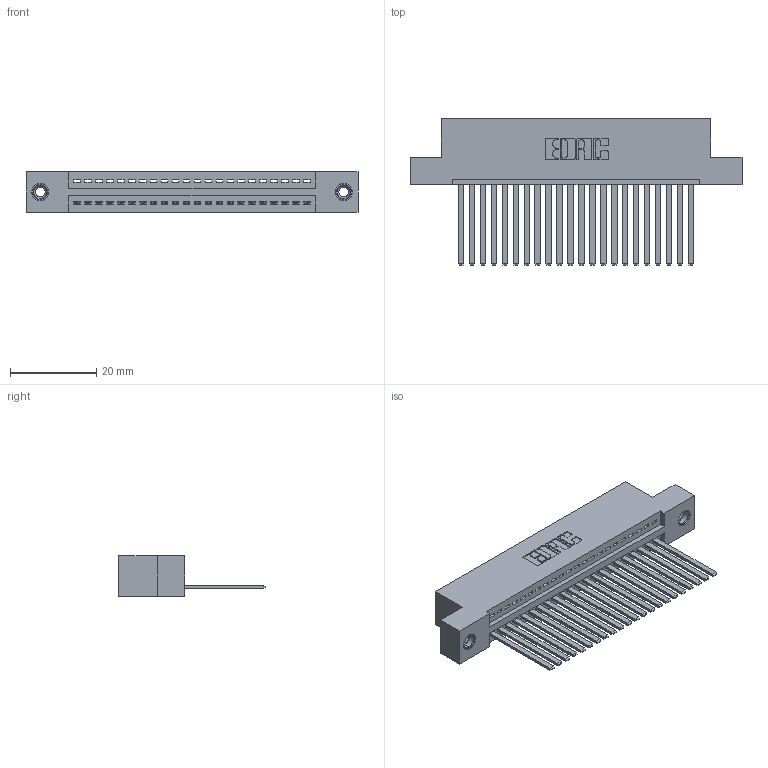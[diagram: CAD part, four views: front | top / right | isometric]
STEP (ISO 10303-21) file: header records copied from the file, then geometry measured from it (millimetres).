
FILE_DESCRIPTION (( 'STEP AP203' ), '1' );
FILE_NAME ('345-022-544-108.STEP', '2019-10-05T00:54:58', ( '' ), ( '' ), 'SwSTEP 2.0', 'SolidWorks 2016', '' );
FILE_SCHEMA (( 'CONFIG_CONTROL_DESIGN' ));
Length unit declared in the file: inch
Products named in the file (4): 345-292-001_345-293-144; 345-250-001_345-250-003-102; 345 Part_Flush Mounting Lugs - 0.156 Dia-TI; 345-022-544-108
Assembly tree (25 placements, depth 2):
  345-022-544-108
    345 Part_Flush Mounting Lugs - 0.156 Dia-TI
    345-292-001_345-293-144  x22
    345-250-001_345-250-003-102  x2
Bounding box: 77.09 x 33.96 x 9.4 mm (x, y, z)
Volume: 7406.4 mm3; surface area: 10354.7 mm2
Topology: 25 solids, 25 shells, 1330 faces, 3953 edges, 2598 vertices
Faces by surface type: plane 904, cylinder 410, cone 12, torus 4
Entity records: 20252 total; most frequent: CARTESIAN_POINT 3489, ORIENTED_EDGE 3438, DIRECTION 3101, EDGE_CURVE 1719, LINE 1483, VECTOR 1483, VERTEX_POINT 1140, AXIS2_PLACEMENT_3D 809
